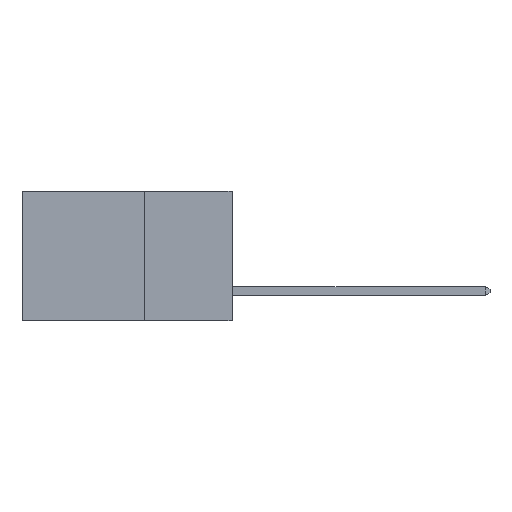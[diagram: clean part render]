
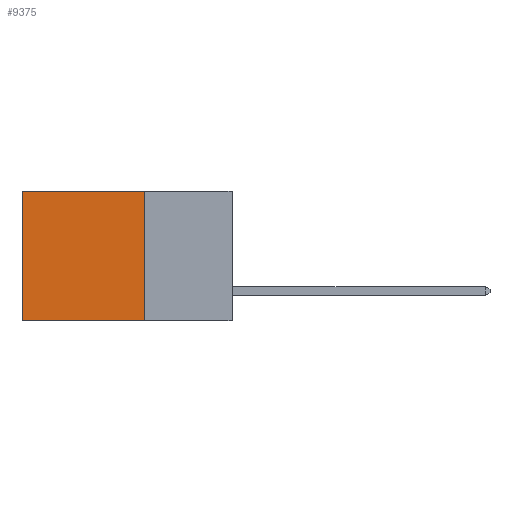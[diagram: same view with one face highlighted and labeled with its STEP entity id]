
A CAD part, left-side view. The second image highlights one B-rep face of the part: STEP entity #9375.
In plain terms, the highlighted planar face has unit normal (-1, 0, 0).
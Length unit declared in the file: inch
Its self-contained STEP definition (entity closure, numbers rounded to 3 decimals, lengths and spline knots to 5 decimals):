
#1275 = CARTESIAN_POINT ( 'NONE',  ( 0.2875, 0.25, 0. ) ) ;
#1434 = ORIENTED_EDGE ( 'NONE', *, *, #18153, .T. ) ;
#2598 = DIRECTION ( 'NONE',  ( 0., 1., 0. ) ) ;
#3362 = DIRECTION ( 'NONE',  ( 1., 0., 0. ) ) ;
#4418 = CARTESIAN_POINT ( 'NONE',  ( 0.2875, 0.25, 0. ) ) ;
#4545 = VERTEX_POINT ( 'NONE', #18873 ) ;
#6319 = DIRECTION ( 'NONE',  ( 0., 0., -1. ) ) ;
#6383 = CARTESIAN_POINT ( 'NONE',  ( 0.2875, 0.25, -0.37 ) ) ;
#7055 = ORIENTED_EDGE ( 'NONE', *, *, #11542, .F. ) ;
#7136 = VECTOR ( 'NONE', #22817, 39.37008 ) ;
#7748 = VECTOR ( 'NONE', #2598, 39.37008 ) ;
#8253 = VERTEX_POINT ( 'NONE', #21421 ) ;
#8417 = EDGE_LOOP ( 'NONE', ( #20773, #7055, #13997, #1434 ) ) ;
#8843 = CARTESIAN_POINT ( 'NONE',  ( 0.2875, 0.6, 0. ) ) ;
#8858 = LINE ( 'NONE', #6383, #7748 ) ;
#8989 = VECTOR ( 'NONE', #22943, 39.37008 ) ;
#9375 = ADVANCED_FACE ( 'NONE', ( #20874 ), #15940, .F. ) ;
#10678 = VECTOR ( 'NONE', #6319, 39.37008 ) ;
#11542 = EDGE_CURVE ( 'NONE', #8253, #13419, #8858, .T. ) ;
#11969 = LINE ( 'NONE', #1275, #7136 ) ;
#13419 = VERTEX_POINT ( 'NONE', #18112 ) ;
#13791 = LINE ( 'NONE', #8843, #8989 ) ;
#13997 = ORIENTED_EDGE ( 'NONE', *, *, #14863, .F. ) ;
#14293 = CARTESIAN_POINT ( 'NONE',  ( 0.2875, 0.25, 0. ) ) ;
#14863 = EDGE_CURVE ( 'NONE', #22426, #8253, #20084, .T. ) ;
#15940 = PLANE ( 'NONE',  #19055 ) ;
#16011 = DIRECTION ( 'NONE',  ( 0., 0., -1. ) ) ;
#18112 = CARTESIAN_POINT ( 'NONE',  ( 0.2875, 0.6, -0.37 ) ) ;
#18153 = EDGE_CURVE ( 'NONE', #22426, #4545, #11969, .T. ) ;
#18873 = CARTESIAN_POINT ( 'NONE',  ( 0.2875, 0.6, 0. ) ) ;
#19055 = AXIS2_PLACEMENT_3D ( 'NONE', #14293, #3362, #16011 ) ;
#19441 = CARTESIAN_POINT ( 'NONE',  ( 0.2875, 0.25, 0. ) ) ;
#20084 = LINE ( 'NONE', #4418, #10678 ) ;
#20352 = EDGE_CURVE ( 'NONE', #4545, #13419, #13791, .T. ) ;
#20773 = ORIENTED_EDGE ( 'NONE', *, *, #20352, .T. ) ;
#20874 = FACE_OUTER_BOUND ( 'NONE', #8417, .T. ) ;
#21421 = CARTESIAN_POINT ( 'NONE',  ( 0.2875, 0.25, -0.37 ) ) ;
#22426 = VERTEX_POINT ( 'NONE', #19441 ) ;
#22817 = DIRECTION ( 'NONE',  ( 0., 1., 0. ) ) ;
#22943 = DIRECTION ( 'NONE',  ( 0., 0., -1. ) ) ;
